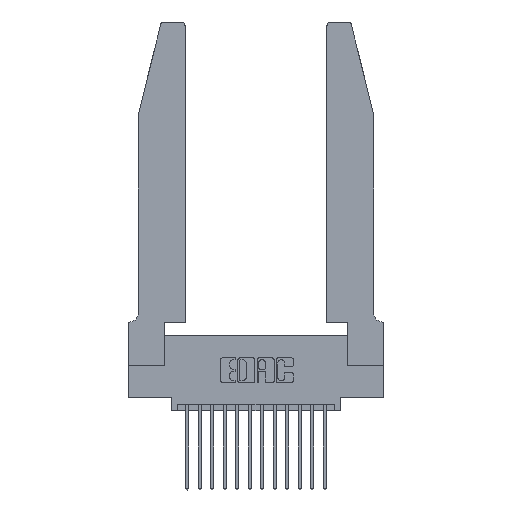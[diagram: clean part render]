
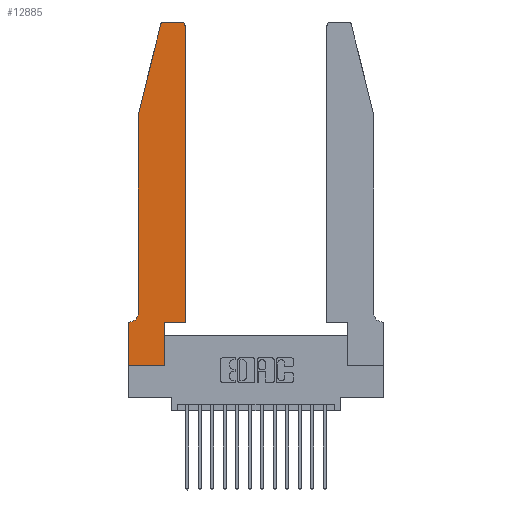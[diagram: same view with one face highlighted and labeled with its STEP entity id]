
A CAD part, top view. The second image highlights one B-rep face of the part: STEP entity #12885.
In plain terms, the highlighted planar face has unit normal (0, 0, 1).
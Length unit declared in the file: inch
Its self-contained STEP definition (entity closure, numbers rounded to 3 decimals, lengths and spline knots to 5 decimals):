
#184 = EDGE_CURVE ( 'NONE', #3860, #6128, #12159, .T. ) ;
#241 = CARTESIAN_POINT ( 'NONE',  ( 0.284, 2.75, 0.37 ) ) ;
#606 = DIRECTION ( 'NONE',  ( 0., -1., 0. ) ) ;
#1047 = CARTESIAN_POINT ( 'NONE',  ( 0.0755, 0.35, 0.37 ) ) ;
#1063 = CARTESIAN_POINT ( 'NONE',  ( 0.2865, 0., 0.37 ) ) ;
#1075 = EDGE_CURVE ( 'NONE', #17795, #11802, #4200, .T. ) ;
#1097 = VECTOR ( 'NONE', #16157, 39.37008 ) ;
#1228 = LINE ( 'NONE', #10291, #14946 ) ;
#1251 = AXIS2_PLACEMENT_3D ( 'NONE', #7147, #11476, #12862 ) ;
#1712 = CARTESIAN_POINT ( 'NONE',  ( 0.4505, 0.35, 0.37 ) ) ;
#1844 = CIRCLE ( 'NONE', #6264, 0.03 ) ;
#2258 = CARTESIAN_POINT ( 'NONE',  ( 0., 0., 0.37 ) ) ;
#2308 = CARTESIAN_POINT ( 'NONE',  ( 0.2605, 2.75, 0.37 ) ) ;
#2405 = VECTOR ( 'NONE', #4440, 39.37008 ) ;
#2600 = VERTEX_POINT ( 'NONE', #1063 ) ;
#2744 = VERTEX_POINT ( 'NONE', #4870 ) ;
#2907 = LINE ( 'NONE', #14387, #13949 ) ;
#3427 = LINE ( 'NONE', #1712, #16477 ) ;
#3495 = FACE_OUTER_BOUND ( 'NONE', #12388, .T. ) ;
#3569 = DIRECTION ( 'NONE',  ( -1., 0., 0. ) ) ;
#3736 = CIRCLE ( 'NONE', #13303, 0.07 ) ;
#3860 = VERTEX_POINT ( 'NONE', #12301 ) ;
#3881 = CARTESIAN_POINT ( 'NONE',  ( 0.284, 2.72, 0.37 ) ) ;
#3914 = CIRCLE ( 'NONE', #14207, 0.03 ) ;
#4152 = VECTOR ( 'NONE', #4955, 39.37008 ) ;
#4200 = LINE ( 'NONE', #2308, #17493 ) ;
#4440 = DIRECTION ( 'NONE',  ( 1., 0., 0. ) ) ;
#4730 = CARTESIAN_POINT ( 'NONE',  ( 0.0755, 2., 0.37 ) ) ;
#4748 = EDGE_CURVE ( 'NONE', #2600, #12676, #2907, .T. ) ;
#4870 = CARTESIAN_POINT ( 'NONE',  ( 0.4505, 0.35, 0.37 ) ) ;
#4955 = DIRECTION ( 'NONE',  ( 0., -1., 0. ) ) ;
#5069 = VECTOR ( 'NONE', #6346, 39.37008 ) ;
#5186 = DIRECTION ( 'NONE',  ( 0., 0., 1. ) ) ;
#5998 = EDGE_CURVE ( 'NONE', #12676, #2744, #8579, .T. ) ;
#6055 = EDGE_CURVE ( 'NONE', #10863, #16286, #12557, .T. ) ;
#6128 = VERTEX_POINT ( 'NONE', #7516 ) ;
#6264 = AXIS2_PLACEMENT_3D ( 'NONE', #17282, #15709, #14459 ) ;
#6346 = DIRECTION ( 'NONE',  ( -0.239, -0.971, 0. ) ) ;
#6660 = CARTESIAN_POINT ( 'NONE',  ( 0.25487, 2.72718, 0.37 ) ) ;
#6665 = ORIENTED_EDGE ( 'NONE', *, *, #9062, .T. ) ;
#6811 = ORIENTED_EDGE ( 'NONE', *, *, #12407, .T. ) ;
#6914 = ORIENTED_EDGE ( 'NONE', *, *, #9593, .T. ) ;
#7147 = CARTESIAN_POINT ( 'NONE',  ( 0., 0.35, 0.37 ) ) ;
#7268 = EDGE_CURVE ( 'NONE', #11802, #10863, #3914, .T. ) ;
#7333 = VECTOR ( 'NONE', #15209, 39.37008 ) ;
#7373 = CARTESIAN_POINT ( 'NONE',  ( 0.4505, 2.72, 0.37 ) ) ;
#7516 = CARTESIAN_POINT ( 'NONE',  ( 0., 0.35, 0.37 ) ) ;
#7933 = ORIENTED_EDGE ( 'NONE', *, *, #12488, .T. ) ;
#8559 = VERTEX_POINT ( 'NONE', #7373 ) ;
#8579 = LINE ( 'NONE', #16091, #1097 ) ;
#8924 = DIRECTION ( 'NONE',  ( 0., 0., -1. ) ) ;
#9062 = EDGE_CURVE ( 'NONE', #16286, #15577, #1228, .T. ) ;
#9068 = ORIENTED_EDGE ( 'NONE', *, *, #1075, .T. ) ;
#9385 = ORIENTED_EDGE ( 'NONE', *, *, #13149, .T. ) ;
#9593 = EDGE_CURVE ( 'NONE', #2744, #8559, #3427, .T. ) ;
#10021 = VERTEX_POINT ( 'NONE', #12361 ) ;
#10168 = CARTESIAN_POINT ( 'NONE',  ( 0.0755, 0.42, 0.37 ) ) ;
#10291 = CARTESIAN_POINT ( 'NONE',  ( 0.0755, 2., 0.37 ) ) ;
#10863 = VERTEX_POINT ( 'NONE', #6660 ) ;
#11106 = ORIENTED_EDGE ( 'NONE', *, *, #6055, .T. ) ;
#11476 = DIRECTION ( 'NONE',  ( 0., 0., 1. ) ) ;
#11630 = LINE ( 'NONE', #2258, #4152 ) ;
#11697 = CARTESIAN_POINT ( 'NONE',  ( 0., 0., 0.37 ) ) ;
#11802 = VERTEX_POINT ( 'NONE', #241 ) ;
#12159 = LINE ( 'NONE', #1047, #7333 ) ;
#12301 = CARTESIAN_POINT ( 'NONE',  ( 0.0055, 0.35, 0.37 ) ) ;
#12361 = CARTESIAN_POINT ( 'NONE',  ( 0., 0., 0.37 ) ) ;
#12388 = EDGE_LOOP ( 'NONE', ( #9068, #14012, #11106, #6665, #7933, #14645, #9385, #6811, #13723, #17608, #6914, #17368 ) ) ;
#12407 = EDGE_CURVE ( 'NONE', #10021, #2600, #15022, .T. ) ;
#12488 = EDGE_CURVE ( 'NONE', #15577, #3860, #3736, .T. ) ;
#12557 = LINE ( 'NONE', #4730, #5069 ) ;
#12676 = VERTEX_POINT ( 'NONE', #18016 ) ;
#12862 = DIRECTION ( 'NONE',  ( 1., 0., 0. ) ) ;
#12877 = DIRECTION ( 'NONE',  ( 0., 1., 0. ) ) ;
#12885 = ADVANCED_FACE ( 'NONE', ( #3495 ), #15613, .T. ) ;
#13149 = EDGE_CURVE ( 'NONE', #6128, #10021, #11630, .T. ) ;
#13250 = CARTESIAN_POINT ( 'NONE',  ( 0.0055, 0.42, 0.37 ) ) ;
#13303 = AXIS2_PLACEMENT_3D ( 'NONE', #13250, #8924, #3569 ) ;
#13594 = CARTESIAN_POINT ( 'NONE',  ( 0.4205, 2.75, 0.37 ) ) ;
#13723 = ORIENTED_EDGE ( 'NONE', *, *, #4748, .T. ) ;
#13949 = VECTOR ( 'NONE', #15819, 39.37008 ) ;
#14012 = ORIENTED_EDGE ( 'NONE', *, *, #7268, .T. ) ;
#14207 = AXIS2_PLACEMENT_3D ( 'NONE', #3881, #5186, #15150 ) ;
#14387 = CARTESIAN_POINT ( 'NONE',  ( 0.2865, 0.35, 0.37 ) ) ;
#14459 = DIRECTION ( 'NONE',  ( 1., 0., 0. ) ) ;
#14645 = ORIENTED_EDGE ( 'NONE', *, *, #184, .T. ) ;
#14946 = VECTOR ( 'NONE', #606, 39.37008 ) ;
#15022 = LINE ( 'NONE', #11697, #2405 ) ;
#15150 = DIRECTION ( 'NONE',  ( 1., 0., 0. ) ) ;
#15209 = DIRECTION ( 'NONE',  ( -1., 0., 0. ) ) ;
#15544 = EDGE_CURVE ( 'NONE', #8559, #17795, #1844, .T. ) ;
#15577 = VERTEX_POINT ( 'NONE', #10168 ) ;
#15613 = PLANE ( 'NONE',  #1251 ) ;
#15709 = DIRECTION ( 'NONE',  ( 0., 0., 1. ) ) ;
#15819 = DIRECTION ( 'NONE',  ( 0., 1., 0. ) ) ;
#16091 = CARTESIAN_POINT ( 'NONE',  ( 0.4505, 0.35, 0.37 ) ) ;
#16157 = DIRECTION ( 'NONE',  ( 1., 0., 0. ) ) ;
#16286 = VERTEX_POINT ( 'NONE', #16373 ) ;
#16373 = CARTESIAN_POINT ( 'NONE',  ( 0.0755, 2., 0.37 ) ) ;
#16477 = VECTOR ( 'NONE', #12877, 39.37008 ) ;
#17282 = CARTESIAN_POINT ( 'NONE',  ( 0.4205, 2.72, 0.37 ) ) ;
#17368 = ORIENTED_EDGE ( 'NONE', *, *, #15544, .T. ) ;
#17493 = VECTOR ( 'NONE', #17728, 39.37008 ) ;
#17608 = ORIENTED_EDGE ( 'NONE', *, *, #5998, .T. ) ;
#17728 = DIRECTION ( 'NONE',  ( -1., 0., 0. ) ) ;
#17795 = VERTEX_POINT ( 'NONE', #13594 ) ;
#18016 = CARTESIAN_POINT ( 'NONE',  ( 0.2865, 0.35, 0.37 ) ) ;
